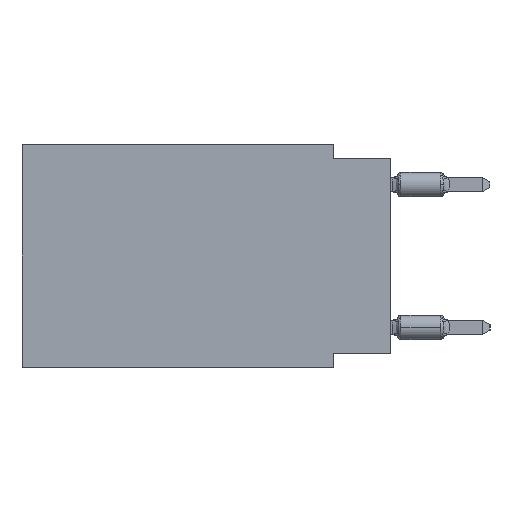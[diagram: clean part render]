
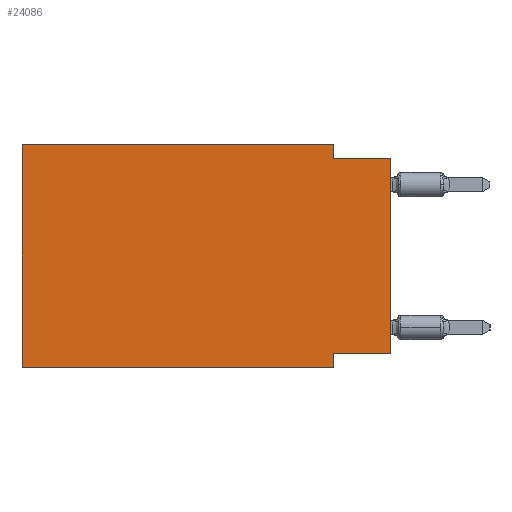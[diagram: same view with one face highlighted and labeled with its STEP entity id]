
A CAD part, left-side view. The second image highlights one B-rep face of the part: STEP entity #24086.
In plain terms, the highlighted planar face has unit normal (-1, 0, 0).
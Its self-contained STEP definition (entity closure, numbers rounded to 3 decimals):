
#725 = VECTOR ( 'NONE', #52186, 1000. ) ;
#1176 = EDGE_CURVE ( 'NONE', #41128, #48004, #9659, .T. ) ;
#1221 = CARTESIAN_POINT ( 'NONE',  ( 0., 2.54, -9.906 ) ) ;
#1386 = VECTOR ( 'NONE', #24368, 1000. ) ;
#2914 = EDGE_CURVE ( 'NONE', #29012, #16163, #54704, .T. ) ;
#3582 = DIRECTION ( 'NONE',  ( 0., 0., -1. ) ) ;
#6267 = ORIENTED_EDGE ( 'NONE', *, *, #18539, .T. ) ;
#6438 = CARTESIAN_POINT ( 'NONE',  ( 0., 0., 0. ) ) ;
#7009 = VERTEX_POINT ( 'NONE', #25565 ) ;
#7140 = CARTESIAN_POINT ( 'NONE',  ( 0., 2.54, 0. ) ) ;
#9591 = LINE ( 'NONE', #32413, #15562 ) ;
#9659 = LINE ( 'NONE', #44182, #725 ) ;
#10073 = LINE ( 'NONE', #10927, #37377 ) ;
#10273 = VERTEX_POINT ( 'NONE', #47454 ) ;
#10509 = AXIS2_PLACEMENT_3D ( 'NONE', #16697, #38109, #3582 ) ;
#10927 = CARTESIAN_POINT ( 'NONE',  ( 0., 0., -9.271 ) ) ;
#14804 = VECTOR ( 'NONE', #48660, 1000. ) ;
#14818 = VERTEX_POINT ( 'NONE', #20422 ) ;
#15562 = VECTOR ( 'NONE', #23299, 1000. ) ;
#15617 = EDGE_CURVE ( 'NONE', #48004, #21856, #28495, .T. ) ;
#15778 = EDGE_CURVE ( 'NONE', #7009, #41128, #9591, .T. ) ;
#15934 = DIRECTION ( 'NONE',  ( 0., -1., 0. ) ) ;
#16027 = EDGE_CURVE ( 'NONE', #14818, #29012, #10073, .T. ) ;
#16163 = VERTEX_POINT ( 'NONE', #1221 ) ;
#16185 = ORIENTED_EDGE ( 'NONE', *, *, #15617, .F. ) ;
#16697 = CARTESIAN_POINT ( 'NONE',  ( 0., 16.383, 0. ) ) ;
#16914 = VECTOR ( 'NONE', #49271, 1000. ) ;
#18539 = EDGE_CURVE ( 'NONE', #14818, #21856, #48943, .T. ) ;
#18896 = ORIENTED_EDGE ( 'NONE', *, *, #15778, .F. ) ;
#20422 = CARTESIAN_POINT ( 'NONE',  ( 0., 0., -9.271 ) ) ;
#21856 = VERTEX_POINT ( 'NONE', #49441 ) ;
#22720 = CARTESIAN_POINT ( 'NONE',  ( 0., 16.383, 0. ) ) ;
#23299 = DIRECTION ( 'NONE',  ( 0., -1., 0. ) ) ;
#24086 = ADVANCED_FACE ( 'NONE', ( #41828 ), #50960, .F. ) ;
#24324 = VECTOR ( 'NONE', #35542, 1000. ) ;
#24368 = DIRECTION ( 'NONE',  ( 0., -1., 0. ) ) ;
#24488 = EDGE_CURVE ( 'NONE', #10273, #16163, #38041, .T. ) ;
#25565 = CARTESIAN_POINT ( 'NONE',  ( 0., 16.383, 0. ) ) ;
#28495 = LINE ( 'NONE', #37613, #55597 ) ;
#29012 = VERTEX_POINT ( 'NONE', #30631 ) ;
#30631 = CARTESIAN_POINT ( 'NONE',  ( 0., 2.54, -9.271 ) ) ;
#32413 = CARTESIAN_POINT ( 'NONE',  ( 0., 16.383, 0. ) ) ;
#32425 = CARTESIAN_POINT ( 'NONE',  ( 0., 2.54, -9.906 ) ) ;
#33560 = ORIENTED_EDGE ( 'NONE', *, *, #24488, .T. ) ;
#34026 = ORIENTED_EDGE ( 'NONE', *, *, #1176, .F. ) ;
#35542 = DIRECTION ( 'NONE',  ( 0., 0., 1. ) ) ;
#37288 = ORIENTED_EDGE ( 'NONE', *, *, #2914, .F. ) ;
#37377 = VECTOR ( 'NONE', #48866, 1000. ) ;
#37613 = CARTESIAN_POINT ( 'NONE',  ( 0., 0., -0.635 ) ) ;
#38041 = LINE ( 'NONE', #50892, #1386 ) ;
#38109 = DIRECTION ( 'NONE',  ( 1., 0., 0. ) ) ;
#41128 = VERTEX_POINT ( 'NONE', #7140 ) ;
#41828 = FACE_OUTER_BOUND ( 'NONE', #49058, .T. ) ;
#42895 = CARTESIAN_POINT ( 'NONE',  ( 0., 2.54, -0.635 ) ) ;
#43443 = ORIENTED_EDGE ( 'NONE', *, *, #16027, .F. ) ;
#44182 = CARTESIAN_POINT ( 'NONE',  ( 0., 2.54, 0. ) ) ;
#47454 = CARTESIAN_POINT ( 'NONE',  ( 0., 16.383, -9.906 ) ) ;
#48004 = VERTEX_POINT ( 'NONE', #42895 ) ;
#48660 = DIRECTION ( 'NONE',  ( 0., 0., 1. ) ) ;
#48866 = DIRECTION ( 'NONE',  ( 0., 1., 0. ) ) ;
#48943 = LINE ( 'NONE', #6438, #14804 ) ;
#49058 = EDGE_LOOP ( 'NONE', ( #6267, #16185, #34026, #18896, #52966, #33560, #37288, #43443 ) ) ;
#49247 = LINE ( 'NONE', #22720, #24324 ) ;
#49271 = DIRECTION ( 'NONE',  ( 0., 0., -1. ) ) ;
#49441 = CARTESIAN_POINT ( 'NONE',  ( 0., 0., -0.635 ) ) ;
#50892 = CARTESIAN_POINT ( 'NONE',  ( 0., 16.383, -9.906 ) ) ;
#50960 = PLANE ( 'NONE',  #10509 ) ;
#52186 = DIRECTION ( 'NONE',  ( 0., 0., -1. ) ) ;
#52966 = ORIENTED_EDGE ( 'NONE', *, *, #54801, .F. ) ;
#54704 = LINE ( 'NONE', #32425, #16914 ) ;
#54801 = EDGE_CURVE ( 'NONE', #10273, #7009, #49247, .T. ) ;
#55597 = VECTOR ( 'NONE', #15934, 1000. ) ;
